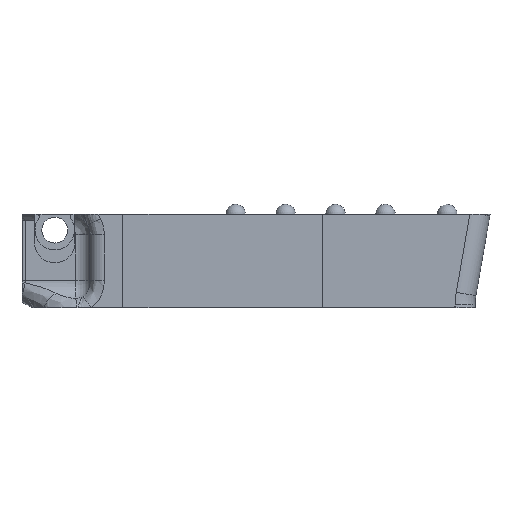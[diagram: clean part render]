
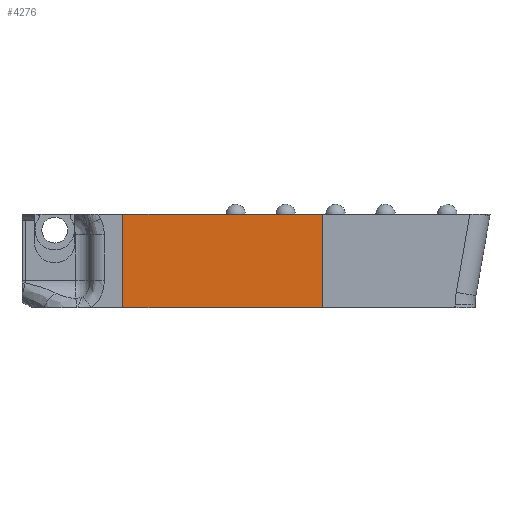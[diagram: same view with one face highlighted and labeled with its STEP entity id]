
A CAD part, front view. The second image highlights one B-rep face of the part: STEP entity #4276.
In plain terms, the highlighted planar face has unit normal (0, -1, 0).
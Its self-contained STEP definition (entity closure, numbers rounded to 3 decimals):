
#24 = ORIENTED_EDGE ( 'NONE', *, *, #2381, .T. ) ;
#25 = PLANE ( 'NONE',  #3825 ) ;
#86 = ORIENTED_EDGE ( 'NONE', *, *, #514, .T. ) ;
#131 = VERTEX_POINT ( 'NONE', #2412 ) ;
#132 = ORIENTED_EDGE ( 'NONE', *, *, #4778, .T. ) ;
#152 = VERTEX_POINT ( 'NONE', #2377 ) ;
#169 = ORIENTED_EDGE ( 'NONE', *, *, #489, .T. ) ;
#364 = CARTESIAN_POINT ( 'NONE',  ( 102.429, -47.207, -5.481 ) ) ;
#489 = EDGE_CURVE ( 'NONE', #1568, #131, #2900, .T. ) ;
#514 = EDGE_CURVE ( 'NONE', #152, #1504, #2839, .T. ) ;
#1344 = LINE ( 'NONE', #4937, #4407 ) ;
#1504 = VERTEX_POINT ( 'NONE', #2161 ) ;
#1568 = VERTEX_POINT ( 'NONE', #2067 ) ;
#1680 = LINE ( 'NONE', #364, #1820 ) ;
#1820 = VECTOR ( 'NONE', #3307, 1000. ) ;
#2067 = CARTESIAN_POINT ( 'NONE',  ( 142.429, -47.207, -5.481 ) ) ;
#2161 = CARTESIAN_POINT ( 'NONE',  ( 102.429, -47.207, -5.481 ) ) ;
#2377 = CARTESIAN_POINT ( 'NONE',  ( 102.429, -47.207, 13.231 ) ) ;
#2381 = EDGE_CURVE ( 'NONE', #131, #152, #1344, .T. ) ;
#2412 = CARTESIAN_POINT ( 'NONE',  ( 142.429, -47.207, 13.231 ) ) ;
#2427 = EDGE_LOOP ( 'NONE', ( #24, #86, #132, #169 ) ) ;
#2783 = VECTOR ( 'NONE', #4662, 1000. ) ;
#2839 = LINE ( 'NONE', #4666, #2783 ) ;
#2895 = VECTOR ( 'NONE', #4758, 1000. ) ;
#2900 = LINE ( 'NONE', #4793, #2895 ) ;
#3307 = DIRECTION ( 'NONE',  ( 1., 0., 0. ) ) ;
#3621 = FACE_OUTER_BOUND ( 'NONE', #2427, .T. ) ;
#3825 = AXIS2_PLACEMENT_3D ( 'NONE', #5012, #4800, #4775 ) ;
#4276 = ADVANCED_FACE ( 'NONE', ( #3621 ), #25, .T. ) ;
#4407 = VECTOR ( 'NONE', #4933, 1000. ) ;
#4662 = DIRECTION ( 'NONE',  ( 0., 0., -1. ) ) ;
#4666 = CARTESIAN_POINT ( 'NONE',  ( 102.429, -47.207, 13.231 ) ) ;
#4758 = DIRECTION ( 'NONE',  ( 0., 0., 1. ) ) ;
#4775 = DIRECTION ( 'NONE',  ( 0., 0., -1. ) ) ;
#4778 = EDGE_CURVE ( 'NONE', #1504, #1568, #1680, .T. ) ;
#4793 = CARTESIAN_POINT ( 'NONE',  ( 142.429, -47.207, -5.481 ) ) ;
#4800 = DIRECTION ( 'NONE',  ( 0., -1., 0. ) ) ;
#4933 = DIRECTION ( 'NONE',  ( -1., 0., 0. ) ) ;
#4937 = CARTESIAN_POINT ( 'NONE',  ( 142.429, -47.207, 13.231 ) ) ;
#5012 = CARTESIAN_POINT ( 'NONE',  ( 0., -47.207, 0. ) ) ;
